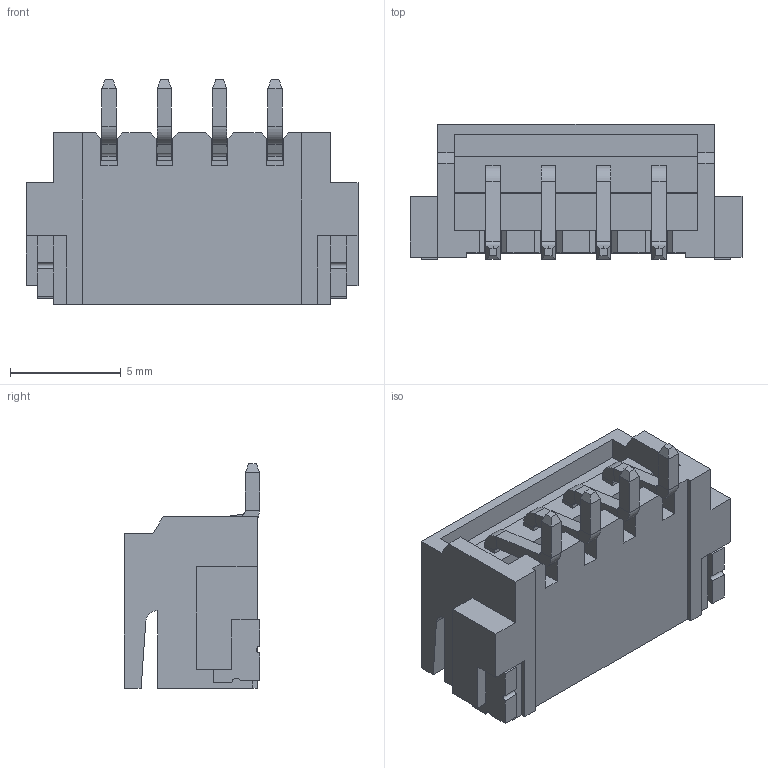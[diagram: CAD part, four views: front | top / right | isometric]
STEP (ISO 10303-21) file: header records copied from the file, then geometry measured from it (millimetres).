
FILE_DESCRIPTION (( 'STEP AP203' ), '1' );
FILE_NAME ('14K-504-418TAA1.STEP', '2024-02-22T13:16:47', ( '' ), ( '' ), 'SwSTEP 2.0', 'SolidWorks 2023', '' );
FILE_SCHEMA (( 'CONFIG_CONTROL_DESIGN' ));
Length unit declared in the file: millimetre
Products named in the file (3): 14K Series SMT Side Entry Insulator_504; 14K Series SMT Pin_Side Entry; 14K-504-418TAA1
Assembly tree (5 placements, depth 2):
  14K-504-418TAA1
    14K Series SMT Side Entry Insulator_504
    14K Series SMT Pin_Side Entry  x4
Bounding box: 15 x 6.1 x 10.15 mm (x, y, z)
Volume: 270.7 mm3; surface area: 827.7 mm2
Topology: 5 solids, 5 shells, 293 faces, 737 edges, 454 vertices
Faces by surface type: plane 262, cylinder 31
Entity records: 6508 total; most frequent: CARTESIAN_POINT 1090, ORIENTED_EDGE 1078, DIRECTION 987, EDGE_CURVE 539, VECTOR 501, LINE 501, VERTEX_POINT 346, AXIS2_PLACEMENT_3D 243
